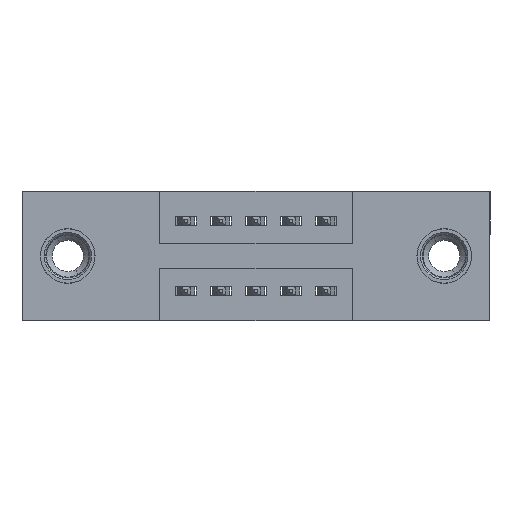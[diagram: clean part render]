
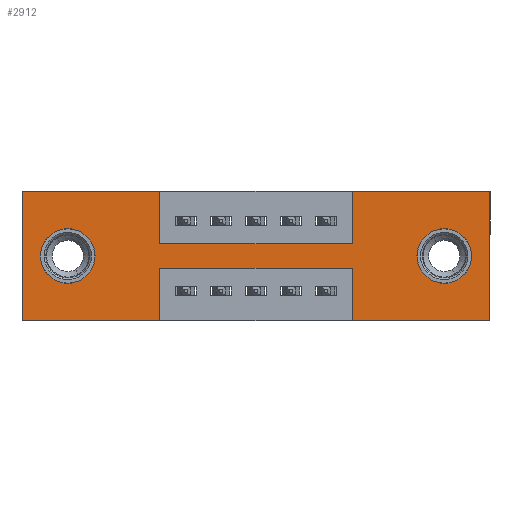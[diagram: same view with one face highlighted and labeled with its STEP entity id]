
A CAD part, front view. The second image highlights one B-rep face of the part: STEP entity #2912.
In plain terms, the highlighted planar face has unit normal (0, -1, 0).
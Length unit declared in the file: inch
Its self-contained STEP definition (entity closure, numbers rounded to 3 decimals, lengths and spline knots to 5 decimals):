
#46 = CARTESIAN_POINT ( 'NONE',  ( 0., 0., 0. ) ) ;
#100 = EDGE_LOOP ( 'NONE', ( #9542, #8863 ) ) ;
#182 = FACE_BOUND ( 'NONE', #5342, .T. ) ;
#186 = DIRECTION ( 'NONE',  ( 0., 0., 1. ) ) ;
#513 = ORIENTED_EDGE ( 'NONE', *, *, #3881, .F. ) ;
#514 = FACE_OUTER_BOUND ( 'NONE', #4485, .T. ) ;
#669 = CARTESIAN_POINT ( 'NONE',  ( 0.3925, 0., -0.22 ) ) ;
#860 = VERTEX_POINT ( 'NONE', #5266 ) ;
#881 = LINE ( 'NONE', #3124, #9078 ) ;
#959 = VERTEX_POINT ( 'NONE', #13520 ) ;
#1148 = CARTESIAN_POINT ( 'NONE',  ( 1.205, 0., -0.107 ) ) ;
#1205 = DIRECTION ( 'NONE',  ( 0., 1., 0. ) ) ;
#1239 = DIRECTION ( 'NONE',  ( -1., 0., 0. ) ) ;
#1268 = VERTEX_POINT ( 'NONE', #669 ) ;
#1419 = VECTOR ( 'NONE', #3529, 39.37008 ) ;
#1454 = ORIENTED_EDGE ( 'NONE', *, *, #3548, .F. ) ;
#1459 = ORIENTED_EDGE ( 'NONE', *, *, #3020, .F. ) ;
#1653 = EDGE_CURVE ( 'NONE', #2486, #860, #3238, .T. ) ;
#1748 = VECTOR ( 'NONE', #1239, 39.37008 ) ;
#1904 = LINE ( 'NONE', #3898, #7255 ) ;
#1961 = CARTESIAN_POINT ( 'NONE',  ( 0.13, 0., -0.263 ) ) ;
#1998 = LINE ( 'NONE', #10457, #12581 ) ;
#2236 = DIRECTION ( 'NONE',  ( 0., 0., -1. ) ) ;
#2239 = DIRECTION ( 'NONE',  ( 0., 1., 0. ) ) ;
#2247 = LINE ( 'NONE', #3846, #4776 ) ;
#2253 = CARTESIAN_POINT ( 'NONE',  ( 1.205, 0., -0.185 ) ) ;
#2401 = ORIENTED_EDGE ( 'NONE', *, *, #12533, .F. ) ;
#2428 = CARTESIAN_POINT ( 'NONE',  ( 0.3925, 0., -0.15 ) ) ;
#2457 = CARTESIAN_POINT ( 'NONE',  ( 0.3925, 0., -0.22 ) ) ;
#2486 = VERTEX_POINT ( 'NONE', #7479 ) ;
#2615 = DIRECTION ( 'NONE',  ( 1., 0., 0. ) ) ;
#2678 = CARTESIAN_POINT ( 'NONE',  ( 0.9425, 0., -0.22 ) ) ;
#2766 = DIRECTION ( 'NONE',  ( 0., 0., 1. ) ) ;
#2791 = ORIENTED_EDGE ( 'NONE', *, *, #10354, .T. ) ;
#2912 = ADVANCED_FACE ( 'NONE', ( #8370, #182, #514 ), #11857, .T. ) ;
#3020 = EDGE_CURVE ( 'NONE', #959, #4145, #12920, .T. ) ;
#3065 = EDGE_CURVE ( 'NONE', #9334, #10120, #4549, .T. ) ;
#3124 = CARTESIAN_POINT ( 'NONE',  ( 1.335, 0., 0. ) ) ;
#3142 = CARTESIAN_POINT ( 'NONE',  ( 0.9425, 0., 0. ) ) ;
#3183 = LINE ( 'NONE', #9549, #3521 ) ;
#3216 = ORIENTED_EDGE ( 'NONE', *, *, #9484, .F. ) ;
#3238 = LINE ( 'NONE', #4235, #11661 ) ;
#3353 = LINE ( 'NONE', #11946, #11431 ) ;
#3396 = CARTESIAN_POINT ( 'NONE',  ( 0., 0., 0. ) ) ;
#3415 = VECTOR ( 'NONE', #10574, 39.37008 ) ;
#3521 = VECTOR ( 'NONE', #10060, 39.37008 ) ;
#3529 = DIRECTION ( 'NONE',  ( 1., 0., 0. ) ) ;
#3548 = EDGE_CURVE ( 'NONE', #4649, #4734, #1998, .T. ) ;
#3662 = EDGE_CURVE ( 'NONE', #10437, #959, #3183, .T. ) ;
#3665 = DIRECTION ( 'NONE',  ( 0., 1., 0. ) ) ;
#3846 = CARTESIAN_POINT ( 'NONE',  ( 0.9425, 0., -0.37 ) ) ;
#3881 = EDGE_CURVE ( 'NONE', #1268, #4649, #3353, .T. ) ;
#3898 = CARTESIAN_POINT ( 'NONE',  ( 0.9425, 0., 0. ) ) ;
#4145 = VERTEX_POINT ( 'NONE', #11666 ) ;
#4235 = CARTESIAN_POINT ( 'NONE',  ( 0., 0., -0.37 ) ) ;
#4278 = LINE ( 'NONE', #12960, #1419 ) ;
#4485 = EDGE_LOOP ( 'NONE', ( #513, #2401, #11212, #7832, #9765, #9682, #8857, #1459, #6526, #3216, #7851, #1454 ) ) ;
#4549 = CIRCLE ( 'NONE', #10512, 0.078 ) ;
#4649 = VERTEX_POINT ( 'NONE', #10304 ) ;
#4734 = VERTEX_POINT ( 'NONE', #6245 ) ;
#4776 = VECTOR ( 'NONE', #2766, 39.37008 ) ;
#4873 = AXIS2_PLACEMENT_3D ( 'NONE', #11902, #11826, #11811 ) ;
#4894 = CARTESIAN_POINT ( 'NONE',  ( 1.335, 0., 0. ) ) ;
#4911 = LINE ( 'NONE', #3396, #12941 ) ;
#4989 = DIRECTION ( 'NONE',  ( 0., 0., 1. ) ) ;
#5058 = EDGE_CURVE ( 'NONE', #10120, #9334, #8176, .T. ) ;
#5144 = VERTEX_POINT ( 'NONE', #2678 ) ;
#5266 = CARTESIAN_POINT ( 'NONE',  ( 0.9425, 0., -0.37 ) ) ;
#5342 = EDGE_LOOP ( 'NONE', ( #2791, #7237 ) ) ;
#5374 = DIRECTION ( 'NONE',  ( -1., 0., 0. ) ) ;
#5515 = VERTEX_POINT ( 'NONE', #46 ) ;
#5551 = DIRECTION ( 'NONE',  ( 0., 0., 1. ) ) ;
#5593 = CIRCLE ( 'NONE', #7992, 0.078 ) ;
#5723 = VERTEX_POINT ( 'NONE', #6823 ) ;
#6245 = CARTESIAN_POINT ( 'NONE',  ( 0., 0., -0.37 ) ) ;
#6246 = LINE ( 'NONE', #9546, #3415 ) ;
#6526 = ORIENTED_EDGE ( 'NONE', *, *, #3662, .F. ) ;
#6600 = DIRECTION ( 'NONE',  ( 0., 1., 0. ) ) ;
#6823 = CARTESIAN_POINT ( 'NONE',  ( 0.13, 0., -0.107 ) ) ;
#7115 = VERTEX_POINT ( 'NONE', #1961 ) ;
#7237 = ORIENTED_EDGE ( 'NONE', *, *, #7302, .T. ) ;
#7255 = VECTOR ( 'NONE', #4989, 39.37008 ) ;
#7302 = EDGE_CURVE ( 'NONE', #7115, #5723, #10595, .T. ) ;
#7479 = CARTESIAN_POINT ( 'NONE',  ( 1.335, 0., -0.37 ) ) ;
#7596 = CARTESIAN_POINT ( 'NONE',  ( 0.13, 0., -0.185 ) ) ;
#7832 = ORIENTED_EDGE ( 'NONE', *, *, #1653, .F. ) ;
#7851 = ORIENTED_EDGE ( 'NONE', *, *, #10950, .F. ) ;
#7992 = AXIS2_PLACEMENT_3D ( 'NONE', #7596, #1205, #8673 ) ;
#8176 = CIRCLE ( 'NONE', #8976, 0.078 ) ;
#8370 = FACE_BOUND ( 'NONE', #100, .T. ) ;
#8444 = DIRECTION ( 'NONE',  ( 0., 0., -1. ) ) ;
#8673 = DIRECTION ( 'NONE',  ( 0., 0., 1. ) ) ;
#8770 = CARTESIAN_POINT ( 'NONE',  ( 0.3925, 0., 0. ) ) ;
#8857 = ORIENTED_EDGE ( 'NONE', *, *, #13251, .F. ) ;
#8863 = ORIENTED_EDGE ( 'NONE', *, *, #5058, .T. ) ;
#8976 = AXIS2_PLACEMENT_3D ( 'NONE', #10029, #3665, #11056 ) ;
#9078 = VECTOR ( 'NONE', #8444, 39.37008 ) ;
#9334 = VERTEX_POINT ( 'NONE', #1148 ) ;
#9484 = EDGE_CURVE ( 'NONE', #5515, #10437, #4278, .T. ) ;
#9542 = ORIENTED_EDGE ( 'NONE', *, *, #3065, .T. ) ;
#9546 = CARTESIAN_POINT ( 'NONE',  ( 0., 0., 0. ) ) ;
#9549 = CARTESIAN_POINT ( 'NONE',  ( 0.3925, 0., 0. ) ) ;
#9682 = ORIENTED_EDGE ( 'NONE', *, *, #10299, .F. ) ;
#9693 = EDGE_CURVE ( 'NONE', #860, #5144, #2247, .T. ) ;
#9765 = ORIENTED_EDGE ( 'NONE', *, *, #10270, .F. ) ;
#9858 = VECTOR ( 'NONE', #2615, 39.37008 ) ;
#9947 = VERTEX_POINT ( 'NONE', #3142 ) ;
#10029 = CARTESIAN_POINT ( 'NONE',  ( 1.205, 0., -0.185 ) ) ;
#10060 = DIRECTION ( 'NONE',  ( 0., 0., -1. ) ) ;
#10120 = VERTEX_POINT ( 'NONE', #10814 ) ;
#10244 = LINE ( 'NONE', #2457, #1748 ) ;
#10270 = EDGE_CURVE ( 'NONE', #13683, #2486, #881, .T. ) ;
#10299 = EDGE_CURVE ( 'NONE', #9947, #13683, #6246, .T. ) ;
#10304 = CARTESIAN_POINT ( 'NONE',  ( 0.3925, 0., -0.37 ) ) ;
#10354 = EDGE_CURVE ( 'NONE', #5723, #7115, #5593, .T. ) ;
#10437 = VERTEX_POINT ( 'NONE', #8770 ) ;
#10445 = DIRECTION ( 'NONE',  ( -1., 0., 0. ) ) ;
#10457 = CARTESIAN_POINT ( 'NONE',  ( 0., 0., -0.37 ) ) ;
#10512 = AXIS2_PLACEMENT_3D ( 'NONE', #2253, #2239, #2236 ) ;
#10574 = DIRECTION ( 'NONE',  ( 1., 0., 0. ) ) ;
#10595 = CIRCLE ( 'NONE', #11321, 0.078 ) ;
#10814 = CARTESIAN_POINT ( 'NONE',  ( 1.205, 0., -0.263 ) ) ;
#10950 = EDGE_CURVE ( 'NONE', #4734, #5515, #4911, .T. ) ;
#11056 = DIRECTION ( 'NONE',  ( 0., 0., -1. ) ) ;
#11212 = ORIENTED_EDGE ( 'NONE', *, *, #9693, .F. ) ;
#11321 = AXIS2_PLACEMENT_3D ( 'NONE', #12862, #6600, #186 ) ;
#11431 = VECTOR ( 'NONE', #13515, 39.37008 ) ;
#11661 = VECTOR ( 'NONE', #5374, 39.37008 ) ;
#11666 = CARTESIAN_POINT ( 'NONE',  ( 0.9425, 0., -0.15 ) ) ;
#11811 = DIRECTION ( 'NONE',  ( 0., 0., -1. ) ) ;
#11826 = DIRECTION ( 'NONE',  ( 0., -1., 0. ) ) ;
#11857 = PLANE ( 'NONE',  #4873 ) ;
#11902 = CARTESIAN_POINT ( 'NONE',  ( 0., 0., -0.37 ) ) ;
#11946 = CARTESIAN_POINT ( 'NONE',  ( 0.3925, 0., -0.37 ) ) ;
#12533 = EDGE_CURVE ( 'NONE', #5144, #1268, #10244, .T. ) ;
#12581 = VECTOR ( 'NONE', #10445, 39.37008 ) ;
#12862 = CARTESIAN_POINT ( 'NONE',  ( 0.13, 0., -0.185 ) ) ;
#12920 = LINE ( 'NONE', #2428, #9858 ) ;
#12941 = VECTOR ( 'NONE', #5551, 39.37008 ) ;
#12960 = CARTESIAN_POINT ( 'NONE',  ( 0., 0., 0. ) ) ;
#13251 = EDGE_CURVE ( 'NONE', #4145, #9947, #1904, .T. ) ;
#13515 = DIRECTION ( 'NONE',  ( 0., 0., -1. ) ) ;
#13520 = CARTESIAN_POINT ( 'NONE',  ( 0.3925, 0., -0.15 ) ) ;
#13683 = VERTEX_POINT ( 'NONE', #4894 ) ;
